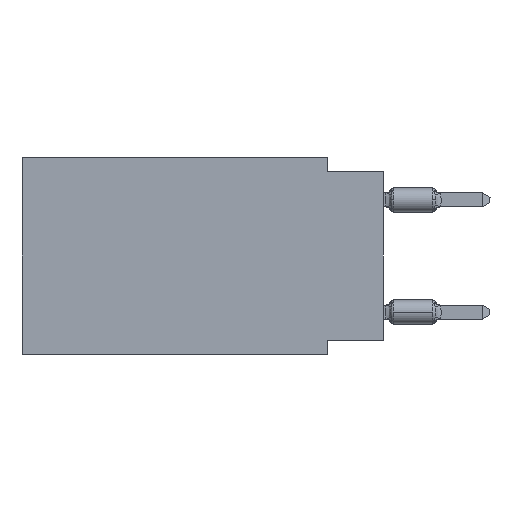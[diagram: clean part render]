
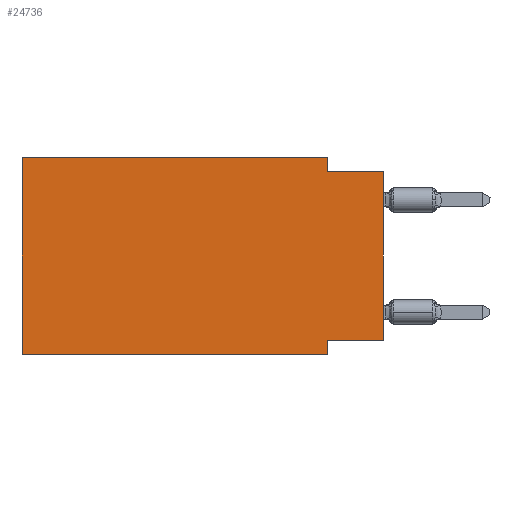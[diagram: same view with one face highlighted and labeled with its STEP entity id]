
A CAD part, left-side view. The second image highlights one B-rep face of the part: STEP entity #24736.
In plain terms, the highlighted planar face has unit normal (-1, 0, 0).
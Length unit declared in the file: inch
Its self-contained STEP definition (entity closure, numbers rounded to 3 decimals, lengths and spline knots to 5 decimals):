
#1912 = CARTESIAN_POINT ( 'NONE',  ( 0., 0.1, -0.35 ) ) ;
#2070 = VERTEX_POINT ( 'NONE', #9802 ) ;
#2153 = DIRECTION ( 'NONE',  ( 0., 0., 1. ) ) ;
#2494 = EDGE_CURVE ( 'NONE', #18069, #47326, #16323, .T. ) ;
#2532 = DIRECTION ( 'NONE',  ( 0., 0., -1. ) ) ;
#3103 = ORIENTED_EDGE ( 'NONE', *, *, #2494, .T. ) ;
#3276 = EDGE_CURVE ( 'NONE', #2070, #14180, #3447, .T. ) ;
#3309 = ORIENTED_EDGE ( 'NONE', *, *, #45387, .F. ) ;
#3447 = LINE ( 'NONE', #32253, #48999 ) ;
#3636 = EDGE_CURVE ( 'NONE', #3673, #47326, #5911, .T. ) ;
#3673 = VERTEX_POINT ( 'NONE', #22522 ) ;
#5094 = LINE ( 'NONE', #46314, #9257 ) ;
#5110 = ORIENTED_EDGE ( 'NONE', *, *, #3636, .F. ) ;
#5524 = DIRECTION ( 'NONE',  ( 0., 0., -1. ) ) ;
#5911 = LINE ( 'NONE', #48497, #12852 ) ;
#7130 = ORIENTED_EDGE ( 'NONE', *, *, #54141, .F. ) ;
#7510 = DIRECTION ( 'NONE',  ( 0., 0., -1. ) ) ;
#7983 = DIRECTION ( 'NONE',  ( 0., 0., 1. ) ) ;
#8263 = CARTESIAN_POINT ( 'NONE',  ( 0., 0., 0. ) ) ;
#9257 = VECTOR ( 'NONE', #29741, 39.37008 ) ;
#9802 = CARTESIAN_POINT ( 'NONE',  ( 0., 0.645, -0.35 ) ) ;
#10728 = CARTESIAN_POINT ( 'NONE',  ( 0., 0.645, 0. ) ) ;
#11949 = PLANE ( 'NONE',  #31916 ) ;
#12852 = VECTOR ( 'NONE', #22809, 39.37008 ) ;
#12909 = LINE ( 'NONE', #46638, #45211 ) ;
#14180 = VERTEX_POINT ( 'NONE', #29567 ) ;
#15539 = VERTEX_POINT ( 'NONE', #35101 ) ;
#16323 = LINE ( 'NONE', #8263, #48303 ) ;
#16472 = DIRECTION ( 'NONE',  ( 0., -1., 0. ) ) ;
#18069 = VERTEX_POINT ( 'NONE', #41118 ) ;
#18735 = ORIENTED_EDGE ( 'NONE', *, *, #29315, .F. ) ;
#20263 = CARTESIAN_POINT ( 'NONE',  ( 0., 0.645, 0. ) ) ;
#21474 = DIRECTION ( 'NONE',  ( 0., -1., 0. ) ) ;
#22522 = CARTESIAN_POINT ( 'NONE',  ( 0., 0.1, -0.025 ) ) ;
#22809 = DIRECTION ( 'NONE',  ( 0., -1., 0. ) ) ;
#23028 = LINE ( 'NONE', #52058, #49540 ) ;
#23203 = LINE ( 'NONE', #10728, #29996 ) ;
#24736 = ADVANCED_FACE ( 'NONE', ( #45406 ), #11949, .F. ) ;
#25720 = ORIENTED_EDGE ( 'NONE', *, *, #3276, .T. ) ;
#26012 = CARTESIAN_POINT ( 'NONE',  ( 0., 0.1, -0.325 ) ) ;
#27783 = EDGE_CURVE ( 'NONE', #2070, #15539, #23203, .T. ) ;
#29315 = EDGE_CURVE ( 'NONE', #45613, #14180, #39855, .T. ) ;
#29567 = CARTESIAN_POINT ( 'NONE',  ( 0., 0.1, -0.35 ) ) ;
#29741 = DIRECTION ( 'NONE',  ( 0., 1., 0. ) ) ;
#29996 = VECTOR ( 'NONE', #2153, 39.37008 ) ;
#31916 = AXIS2_PLACEMENT_3D ( 'NONE', #20263, #49822, #7510 ) ;
#32253 = CARTESIAN_POINT ( 'NONE',  ( 0., 0.645, -0.35 ) ) ;
#34193 = ORIENTED_EDGE ( 'NONE', *, *, #35188, .F. ) ;
#35101 = CARTESIAN_POINT ( 'NONE',  ( 0., 0.645, 0. ) ) ;
#35188 = EDGE_CURVE ( 'NONE', #15539, #41323, #12909, .T. ) ;
#39855 = LINE ( 'NONE', #1912, #51701 ) ;
#41118 = CARTESIAN_POINT ( 'NONE',  ( 0., 0., -0.325 ) ) ;
#41323 = VERTEX_POINT ( 'NONE', #50421 ) ;
#45211 = VECTOR ( 'NONE', #21474, 39.37008 ) ;
#45387 = EDGE_CURVE ( 'NONE', #41323, #3673, #23028, .T. ) ;
#45406 = FACE_OUTER_BOUND ( 'NONE', #54543, .T. ) ;
#45613 = VERTEX_POINT ( 'NONE', #26012 ) ;
#46314 = CARTESIAN_POINT ( 'NONE',  ( 0., 0., -0.325 ) ) ;
#46638 = CARTESIAN_POINT ( 'NONE',  ( 0., 0.645, 0. ) ) ;
#47213 = CARTESIAN_POINT ( 'NONE',  ( 0., 0., -0.025 ) ) ;
#47326 = VERTEX_POINT ( 'NONE', #47213 ) ;
#48303 = VECTOR ( 'NONE', #7983, 39.37008 ) ;
#48497 = CARTESIAN_POINT ( 'NONE',  ( 0., 0., -0.025 ) ) ;
#48999 = VECTOR ( 'NONE', #16472, 39.37008 ) ;
#49540 = VECTOR ( 'NONE', #2532, 39.37008 ) ;
#49822 = DIRECTION ( 'NONE',  ( 1., 0., 0. ) ) ;
#50421 = CARTESIAN_POINT ( 'NONE',  ( 0., 0.1, 0. ) ) ;
#51701 = VECTOR ( 'NONE', #5524, 39.37008 ) ;
#52058 = CARTESIAN_POINT ( 'NONE',  ( 0., 0.1, 0. ) ) ;
#54042 = ORIENTED_EDGE ( 'NONE', *, *, #27783, .F. ) ;
#54141 = EDGE_CURVE ( 'NONE', #18069, #45613, #5094, .T. ) ;
#54543 = EDGE_LOOP ( 'NONE', ( #3103, #5110, #3309, #34193, #54042, #25720, #18735, #7130 ) ) ;
